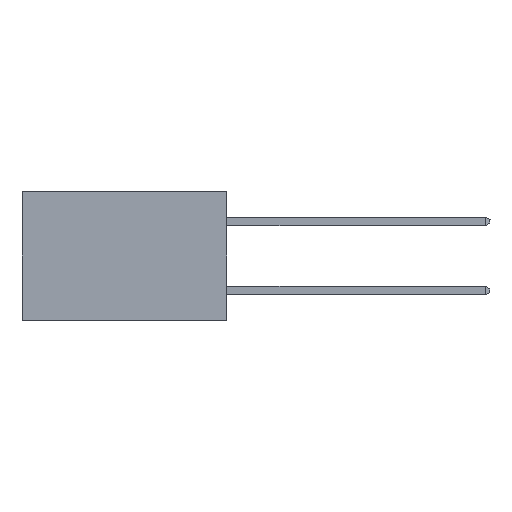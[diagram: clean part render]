
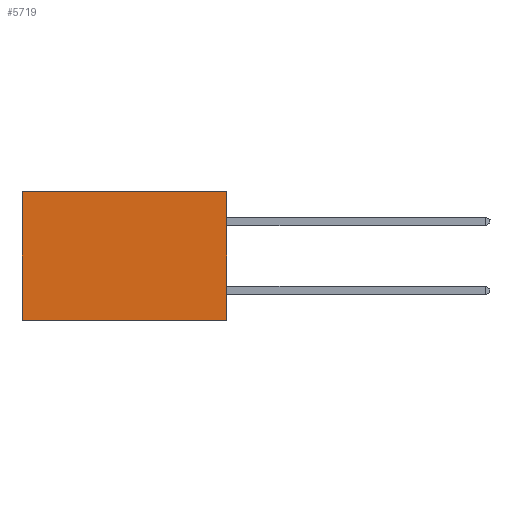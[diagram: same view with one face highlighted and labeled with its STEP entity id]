
A CAD part, left-side view. The second image highlights one B-rep face of the part: STEP entity #5719.
In plain terms, the highlighted planar face has unit normal (-1, 0, 0).
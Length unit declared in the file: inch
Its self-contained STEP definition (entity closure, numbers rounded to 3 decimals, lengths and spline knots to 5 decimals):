
#173 = VERTEX_POINT ( 'NONE', #8858 ) ;
#184 = DIRECTION ( 'NONE',  ( 0., 1., 0. ) ) ;
#511 = DIRECTION ( 'NONE',  ( 0., 0., -1. ) ) ;
#543 = EDGE_CURVE ( 'NONE', #4548, #1876, #7878, .T. ) ;
#550 = ORIENTED_EDGE ( 'NONE', *, *, #9425, .F. ) ;
#789 = CARTESIAN_POINT ( 'NONE',  ( 0.277, 0.59, -0.37 ) ) ;
#1769 = CARTESIAN_POINT ( 'NONE',  ( 0.277, 0., 0. ) ) ;
#1862 = VECTOR ( 'NONE', #8034, 39.37008 ) ;
#1876 = VERTEX_POINT ( 'NONE', #6386 ) ;
#1911 = VECTOR ( 'NONE', #184, 39.37008 ) ;
#2418 = ORIENTED_EDGE ( 'NONE', *, *, #7713, .T. ) ;
#2872 = ORIENTED_EDGE ( 'NONE', *, *, #4321, .T. ) ;
#3210 = AXIS2_PLACEMENT_3D ( 'NONE', #6644, #6605, #6470 ) ;
#3274 = VECTOR ( 'NONE', #511, 39.37008 ) ;
#3504 = LINE ( 'NONE', #789, #3274 ) ;
#3911 = LINE ( 'NONE', #1769, #1911 ) ;
#3920 = CARTESIAN_POINT ( 'NONE',  ( 0.277, 0.59, -0.37 ) ) ;
#3962 = DIRECTION ( 'NONE',  ( 0., 1., 0. ) ) ;
#4180 = VECTOR ( 'NONE', #3962, 39.37008 ) ;
#4321 = EDGE_CURVE ( 'NONE', #4548, #173, #3911, .T. ) ;
#4548 = VERTEX_POINT ( 'NONE', #7862 ) ;
#5719 = ADVANCED_FACE ( 'NONE', ( #6010 ), #7383, .F. ) ;
#6010 = FACE_OUTER_BOUND ( 'NONE', #6675, .T. ) ;
#6290 = LINE ( 'NONE', #7505, #4180 ) ;
#6386 = CARTESIAN_POINT ( 'NONE',  ( 0.277, 0., -0.37 ) ) ;
#6470 = DIRECTION ( 'NONE',  ( 0., 0., -1. ) ) ;
#6605 = DIRECTION ( 'NONE',  ( 1., 0., 0. ) ) ;
#6644 = CARTESIAN_POINT ( 'NONE',  ( 0.277, 0., -0.37 ) ) ;
#6675 = EDGE_LOOP ( 'NONE', ( #2418, #550, #8377, #2872 ) ) ;
#7314 = VERTEX_POINT ( 'NONE', #3920 ) ;
#7383 = PLANE ( 'NONE',  #3210 ) ;
#7505 = CARTESIAN_POINT ( 'NONE',  ( 0.277, 0., -0.37 ) ) ;
#7713 = EDGE_CURVE ( 'NONE', #173, #7314, #3504, .T. ) ;
#7862 = CARTESIAN_POINT ( 'NONE',  ( 0.277, 0., 0. ) ) ;
#7878 = LINE ( 'NONE', #8466, #1862 ) ;
#8034 = DIRECTION ( 'NONE',  ( 0., 0., -1. ) ) ;
#8377 = ORIENTED_EDGE ( 'NONE', *, *, #543, .F. ) ;
#8466 = CARTESIAN_POINT ( 'NONE',  ( 0.277, 0., -0.37 ) ) ;
#8858 = CARTESIAN_POINT ( 'NONE',  ( 0.277, 0.59, 0. ) ) ;
#9425 = EDGE_CURVE ( 'NONE', #1876, #7314, #6290, .T. ) ;
